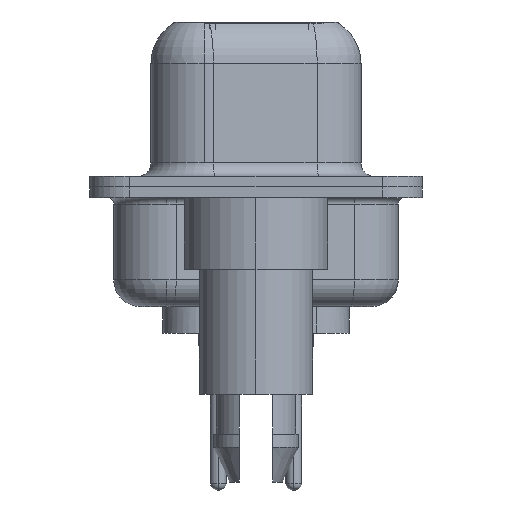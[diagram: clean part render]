
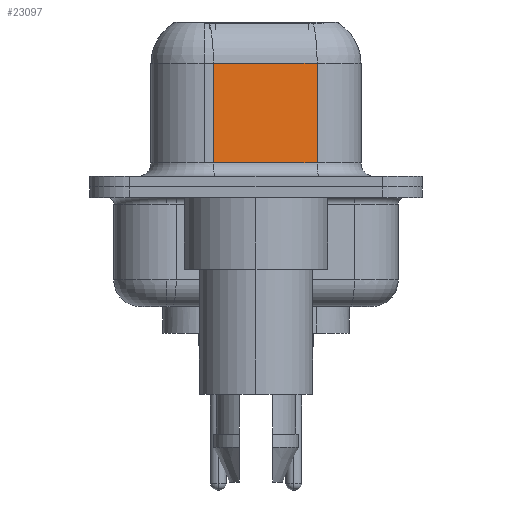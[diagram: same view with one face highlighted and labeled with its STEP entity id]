
A CAD part, left-side view. The second image highlights one B-rep face of the part: STEP entity #23097.
In plain terms, the highlighted planar face has unit normal (-0.985, -0.174, 0).
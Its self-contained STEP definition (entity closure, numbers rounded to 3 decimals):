
#240 = VERTEX_POINT ( 'NONE', #20691 ) ;
#744 = DIRECTION ( 'NONE',  ( -0.174, 0.985, 0. ) ) ;
#2554 = ORIENTED_EDGE ( 'NONE', *, *, #16852, .F. ) ;
#2913 = AXIS2_PLACEMENT_3D ( 'NONE', #27174, #10759, #12584 ) ;
#5046 = CARTESIAN_POINT ( 'NONE',  ( 5.068, -2.297, 4.65 ) ) ;
#5645 = EDGE_CURVE ( 'NONE', #23283, #15569, #18901, .T. ) ;
#6341 = ORIENTED_EDGE ( 'NONE', *, *, #26848, .T. ) ;
#7025 = VECTOR ( 'NONE', #8865, 1000. ) ;
#7063 = ORIENTED_EDGE ( 'NONE', *, *, #18090, .T. ) ;
#8103 = DIRECTION ( 'NONE',  ( 0., 0., -1. ) ) ;
#8409 = VERTEX_POINT ( 'NONE', #14151 ) ;
#8665 = CARTESIAN_POINT ( 'NONE',  ( 4.38, 1.603, 4.65 ) ) ;
#8865 = DIRECTION ( 'NONE',  ( 0.174, -0.985, 0. ) ) ;
#9338 = VECTOR ( 'NONE', #8103, 1000. ) ;
#10345 = CARTESIAN_POINT ( 'NONE',  ( 5.068, -2.297, 6.4 ) ) ;
#10759 = DIRECTION ( 'NONE',  ( 0.985, 0.174, 0. ) ) ;
#12584 = DIRECTION ( 'NONE',  ( -0.174, 0.985, 0. ) ) ;
#13058 = LINE ( 'NONE', #17115, #7025 ) ;
#14151 = CARTESIAN_POINT ( 'NONE',  ( 5.068, -2.297, 0.9 ) ) ;
#14970 = CARTESIAN_POINT ( 'NONE',  ( 4.38, 1.603, 6.4 ) ) ;
#15392 = VECTOR ( 'NONE', #19032, 1000. ) ;
#15487 = ORIENTED_EDGE ( 'NONE', *, *, #5645, .T. ) ;
#15569 = VERTEX_POINT ( 'NONE', #27166 ) ;
#16852 = EDGE_CURVE ( 'NONE', #240, #8409, #27445, .T. ) ;
#17115 = CARTESIAN_POINT ( 'NONE',  ( 5.068, -2.297, 0.9 ) ) ;
#18090 = EDGE_CURVE ( 'NONE', #240, #23283, #19975, .T. ) ;
#18717 = FACE_OUTER_BOUND ( 'NONE', #21922, .T. ) ;
#18901 = LINE ( 'NONE', #14970, #15392 ) ;
#19032 = DIRECTION ( 'NONE',  ( 0., 0., -1. ) ) ;
#19975 = LINE ( 'NONE', #5046, #26713 ) ;
#20691 = CARTESIAN_POINT ( 'NONE',  ( 5.068, -2.297, 4.65 ) ) ;
#21922 = EDGE_LOOP ( 'NONE', ( #2554, #7063, #15487, #6341 ) ) ;
#22882 = PLANE ( 'NONE',  #2913 ) ;
#23097 = ADVANCED_FACE ( 'NONE', ( #18717 ), #22882, .F. ) ;
#23283 = VERTEX_POINT ( 'NONE', #8665 ) ;
#26713 = VECTOR ( 'NONE', #744, 1000. ) ;
#26848 = EDGE_CURVE ( 'NONE', #15569, #8409, #13058, .T. ) ;
#27166 = CARTESIAN_POINT ( 'NONE',  ( 4.38, 1.603, 0.9 ) ) ;
#27174 = CARTESIAN_POINT ( 'NONE',  ( 5.068, -2.297, 6.4 ) ) ;
#27445 = LINE ( 'NONE', #10345, #9338 ) ;
